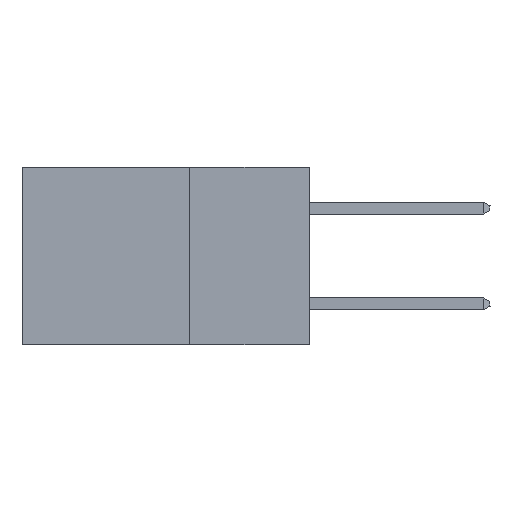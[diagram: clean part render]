
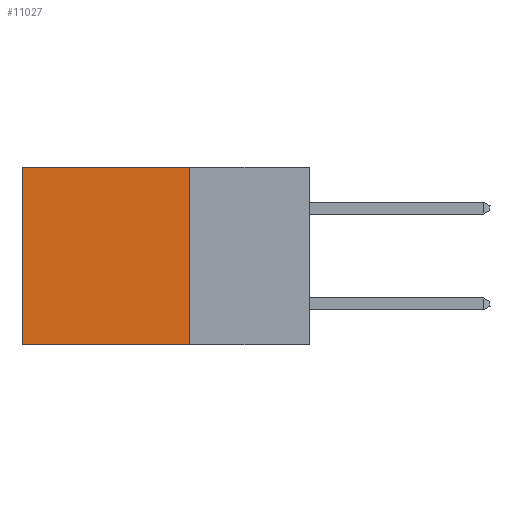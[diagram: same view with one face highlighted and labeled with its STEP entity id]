
A CAD part, left-side view. The second image highlights one B-rep face of the part: STEP entity #11027.
In plain terms, the highlighted planar face has unit normal (-1, 0, 0).
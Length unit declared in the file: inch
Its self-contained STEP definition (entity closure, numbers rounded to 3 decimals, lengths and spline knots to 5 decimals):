
#868 = DIRECTION ( 'NONE',  ( 0., 0., -1. ) ) ;
#1020 = VECTOR ( 'NONE', #19159, 39.37008 ) ;
#1537 = FACE_OUTER_BOUND ( 'NONE', #9120, .T. ) ;
#2677 = ORIENTED_EDGE ( 'NONE', *, *, #26128, .T. ) ;
#3436 = DIRECTION ( 'NONE',  ( 1., 0., 0. ) ) ;
#3639 = CARTESIAN_POINT ( 'NONE',  ( 0.2875, 0.25, 0. ) ) ;
#3770 = ORIENTED_EDGE ( 'NONE', *, *, #5864, .F. ) ;
#4668 = VECTOR ( 'NONE', #17441, 39.37008 ) ;
#4827 = CARTESIAN_POINT ( 'NONE',  ( 0.2875, 0.25, -0.37 ) ) ;
#5756 = LINE ( 'NONE', #15272, #28861 ) ;
#5864 = EDGE_CURVE ( 'NONE', #14537, #16380, #20163, .T. ) ;
#7679 = AXIS2_PLACEMENT_3D ( 'NONE', #24884, #3436, #20199 ) ;
#9120 = EDGE_LOOP ( 'NONE', ( #29044, #3770, #20937, #2677 ) ) ;
#10213 = CARTESIAN_POINT ( 'NONE',  ( 0.2875, 0.25, 0. ) ) ;
#11027 = ADVANCED_FACE ( 'NONE', ( #1537 ), #29621, .F. ) ;
#11033 = LINE ( 'NONE', #10213, #4668 ) ;
#12110 = VECTOR ( 'NONE', #17531, 39.37008 ) ;
#14537 = VERTEX_POINT ( 'NONE', #23213 ) ;
#15272 = CARTESIAN_POINT ( 'NONE',  ( 0.2875, 0.6, 0. ) ) ;
#16380 = VERTEX_POINT ( 'NONE', #25165 ) ;
#17441 = DIRECTION ( 'NONE',  ( 0., 1., 0. ) ) ;
#17531 = DIRECTION ( 'NONE',  ( 0., 0., -1. ) ) ;
#18249 = EDGE_CURVE ( 'NONE', #29541, #16380, #5756, .T. ) ;
#18478 = LINE ( 'NONE', #24612, #12110 ) ;
#19159 = DIRECTION ( 'NONE',  ( 0., 1., 0. ) ) ;
#20163 = LINE ( 'NONE', #4827, #1020 ) ;
#20199 = DIRECTION ( 'NONE',  ( 0., 0., -1. ) ) ;
#20937 = ORIENTED_EDGE ( 'NONE', *, *, #21209, .F. ) ;
#21209 = EDGE_CURVE ( 'NONE', #25661, #14537, #18478, .T. ) ;
#22714 = CARTESIAN_POINT ( 'NONE',  ( 0.2875, 0.6, 0. ) ) ;
#23213 = CARTESIAN_POINT ( 'NONE',  ( 0.2875, 0.25, -0.37 ) ) ;
#24612 = CARTESIAN_POINT ( 'NONE',  ( 0.2875, 0.25, 0. ) ) ;
#24884 = CARTESIAN_POINT ( 'NONE',  ( 0.2875, 0.25, 0. ) ) ;
#25165 = CARTESIAN_POINT ( 'NONE',  ( 0.2875, 0.6, -0.37 ) ) ;
#25661 = VERTEX_POINT ( 'NONE', #3639 ) ;
#26128 = EDGE_CURVE ( 'NONE', #25661, #29541, #11033, .T. ) ;
#28861 = VECTOR ( 'NONE', #868, 39.37008 ) ;
#29044 = ORIENTED_EDGE ( 'NONE', *, *, #18249, .T. ) ;
#29541 = VERTEX_POINT ( 'NONE', #22714 ) ;
#29621 = PLANE ( 'NONE',  #7679 ) ;
